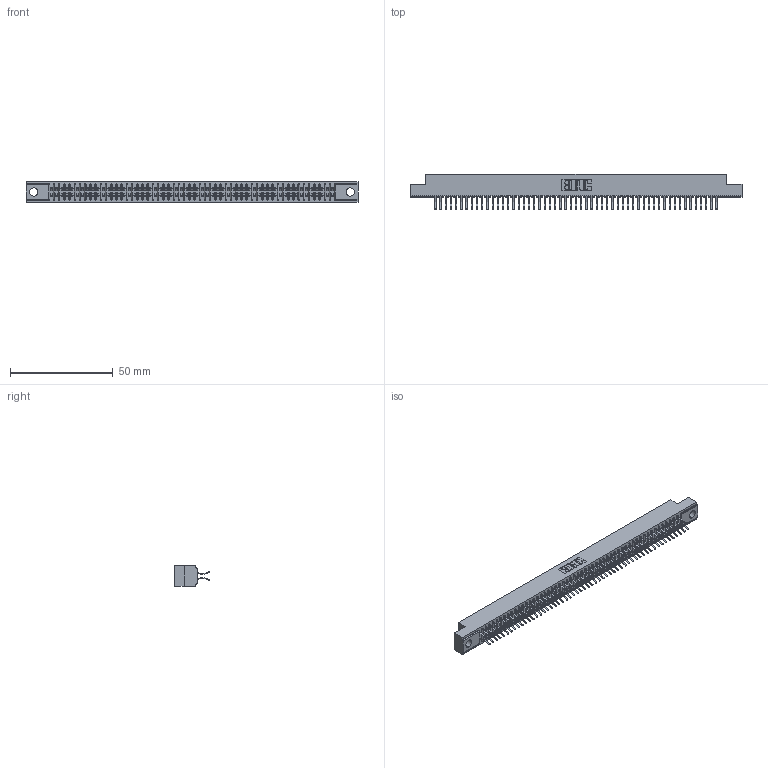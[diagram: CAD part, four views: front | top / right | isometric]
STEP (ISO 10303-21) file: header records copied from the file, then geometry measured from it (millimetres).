
FILE_DESCRIPTION (( 'STEP AP203' ), '1' );
FILE_NAME ('341-110-556-204.STEP', '2018-08-08T12:52:01', ( '' ), ( '' ), 'SwSTEP 2.0', 'SolidWorks 2016', '' );
FILE_SCHEMA (( 'CONFIG_CONTROL_DESIGN' ));
Length unit declared in the file: inch
Products named in the file (3): 341 Part_.156 (3.96) Dia Mounting Holes; 341-292-001_341-292-156; 341-110-556-204
Assembly tree (111 placements, depth 2):
  341-110-556-204
    341 Part_.156 (3.96) Dia Mounting Holes
    341-292-001_341-292-156  x110
Bounding box: 161.93 x 17.07 x 10.16 mm (x, y, z)
Volume: 11897.9 mm3; surface area: 21680.1 mm2
Topology: 111 solids, 111 shells, 7830 faces, 22737 edges, 14750 vertices
Faces by surface type: plane 4482, cylinder 3128, sphere 112, torus 108
Entity records: 65388 total; most frequent: CARTESIAN_POINT 10875, ORIENTED_EDGE 10806, DIRECTION 10541, EDGE_CURVE 5403, VECTOR 4381, LINE 4381, VERTEX_POINT 3414, AXIS2_PLACEMENT_3D 3080
